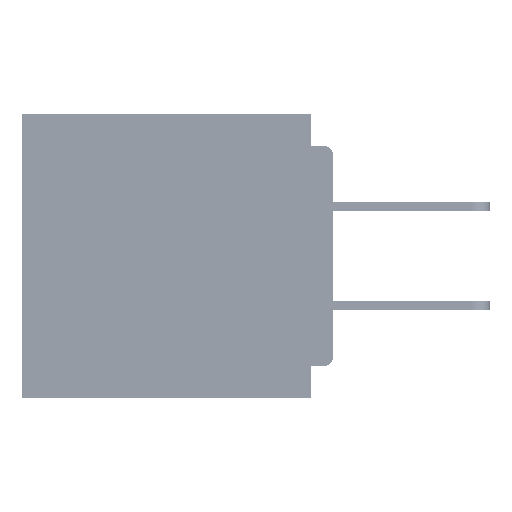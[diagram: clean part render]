
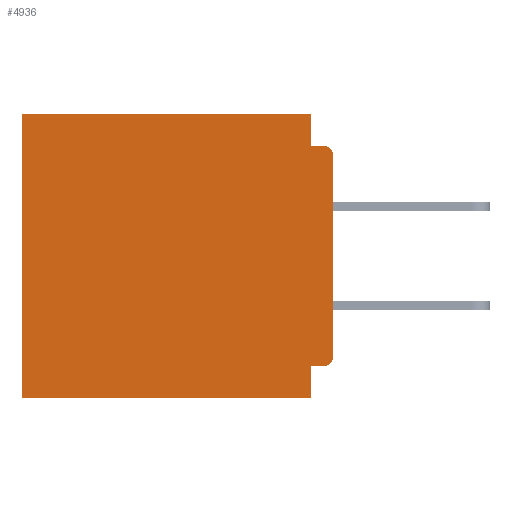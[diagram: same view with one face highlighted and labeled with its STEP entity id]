
A CAD part, left-side view. The second image highlights one B-rep face of the part: STEP entity #4936.
In plain terms, the highlighted planar face has unit normal (-1, 0, 0).
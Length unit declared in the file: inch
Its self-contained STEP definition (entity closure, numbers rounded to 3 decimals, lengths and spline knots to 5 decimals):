
#6 = ORIENTED_EDGE ( 'NONE', *, *, #24385, .F. ) ;
#186 = VERTEX_POINT ( 'NONE', #56536 ) ;
#1119 = VERTEX_POINT ( 'NONE', #56077 ) ;
#1601 = FACE_OUTER_BOUND ( 'NONE', #58669, .T. ) ;
#1822 = VERTEX_POINT ( 'NONE', #17377 ) ;
#1974 = PLANE ( 'NONE',  #14499 ) ;
#2165 = ORIENTED_EDGE ( 'NONE', *, *, #49622, .T. ) ;
#2526 = ORIENTED_EDGE ( 'NONE', *, *, #40947, .F. ) ;
#3678 = CARTESIAN_POINT ( 'NONE',  ( 0.3, 0., 0. ) ) ;
#3712 = AXIS2_PLACEMENT_3D ( 'NONE', #49629, #21771, #54325 ) ;
#3811 = CIRCLE ( 'NONE', #28204, 0.015 ) ;
#4936 = ADVANCED_FACE ( 'NONE', ( #1601 ), #1974, .F. ) ;
#5066 = VERTEX_POINT ( 'NONE', #24203 ) ;
#5212 = VECTOR ( 'NONE', #17366, 39.37008 ) ;
#7191 = ORIENTED_EDGE ( 'NONE', *, *, #28212, .F. ) ;
#7407 = CARTESIAN_POINT ( 'NONE',  ( 0.3, 0.437, 0. ) ) ;
#7862 = DIRECTION ( 'NONE',  ( 0., -1., 0. ) ) ;
#8269 = EDGE_CURVE ( 'NONE', #5066, #24304, #17191, .T. ) ;
#10052 = CIRCLE ( 'NONE', #3712, 0.015 ) ;
#11329 = DIRECTION ( 'NONE',  ( 1., 0., 0. ) ) ;
#12685 = DIRECTION ( 'NONE',  ( -1., 0., 0. ) ) ;
#14499 = AXIS2_PLACEMENT_3D ( 'NONE', #39167, #11329, #43852 ) ;
#16113 = VERTEX_POINT ( 'NONE', #37213 ) ;
#17191 = LINE ( 'NONE', #3678, #52838 ) ;
#17366 = DIRECTION ( 'NONE',  ( 0., 0., -1. ) ) ;
#17377 = CARTESIAN_POINT ( 'NONE',  ( 0.3, 0.031, -0.355 ) ) ;
#17601 = EDGE_CURVE ( 'NONE', #5066, #1119, #39386, .T. ) ;
#17845 = CARTESIAN_POINT ( 'NONE',  ( 0.3, 0., -0.4 ) ) ;
#18385 = VECTOR ( 'NONE', #50360, 39.37008 ) ;
#18921 = CARTESIAN_POINT ( 'NONE',  ( 0.3, 0.437, -0.4 ) ) ;
#19034 = LINE ( 'NONE', #22015, #5212 ) ;
#19107 = LINE ( 'NONE', #21187, #29941 ) ;
#20383 = ORIENTED_EDGE ( 'NONE', *, *, #23775, .F. ) ;
#21187 = CARTESIAN_POINT ( 'NONE',  ( 0.3, 0.437, -0.4 ) ) ;
#21771 = DIRECTION ( 'NONE',  ( -1., 0., 0. ) ) ;
#22015 = CARTESIAN_POINT ( 'NONE',  ( 0.3, 0., -0.4 ) ) ;
#23077 = DIRECTION ( 'NONE',  ( 0., 0., -1. ) ) ;
#23775 = EDGE_CURVE ( 'NONE', #16113, #25872, #40204, .T. ) ;
#24203 = CARTESIAN_POINT ( 'NONE',  ( 0.3, 0.031, 0. ) ) ;
#24304 = VERTEX_POINT ( 'NONE', #7407 ) ;
#24385 = EDGE_CURVE ( 'NONE', #45454, #46795, #19034, .T. ) ;
#25625 = CARTESIAN_POINT ( 'NONE',  ( 0.3, 0., -0.34 ) ) ;
#25872 = VERTEX_POINT ( 'NONE', #18921 ) ;
#27765 = CARTESIAN_POINT ( 'NONE',  ( 0.3, 0.015, -0.355 ) ) ;
#28204 = AXIS2_PLACEMENT_3D ( 'NONE', #40528, #12685, #45212 ) ;
#28212 = EDGE_CURVE ( 'NONE', #1822, #16113, #38984, .T. ) ;
#29413 = DIRECTION ( 'NONE',  ( 0., 0., -1. ) ) ;
#29941 = VECTOR ( 'NONE', #23077, 39.37008 ) ;
#30906 = EDGE_CURVE ( 'NONE', #47703, #46795, #3811, .T. ) ;
#31175 = ORIENTED_EDGE ( 'NONE', *, *, #45833, .T. ) ;
#33935 = CARTESIAN_POINT ( 'NONE',  ( 0.3, 0., -0.355 ) ) ;
#34951 = EDGE_CURVE ( 'NONE', #47703, #1822, #52752, .T. ) ;
#35737 = CARTESIAN_POINT ( 'NONE',  ( 0.3, 0., -0.045 ) ) ;
#37213 = CARTESIAN_POINT ( 'NONE',  ( 0.3, 0.031, -0.4 ) ) ;
#37937 = VECTOR ( 'NONE', #38262, 39.37008 ) ;
#38262 = DIRECTION ( 'NONE',  ( 0., 0., -1. ) ) ;
#38644 = DIRECTION ( 'NONE',  ( 0., 1., 0. ) ) ;
#38903 = VECTOR ( 'NONE', #38644, 39.37008 ) ;
#38984 = LINE ( 'NONE', #57310, #51379 ) ;
#39167 = CARTESIAN_POINT ( 'NONE',  ( 0.3, 0., -0.4 ) ) ;
#39386 = LINE ( 'NONE', #42941, #37937 ) ;
#40204 = LINE ( 'NONE', #17845, #18385 ) ;
#40528 = CARTESIAN_POINT ( 'NONE',  ( 0.3, 0.015, -0.34 ) ) ;
#40947 = EDGE_CURVE ( 'NONE', #1119, #186, #55364, .T. ) ;
#42941 = CARTESIAN_POINT ( 'NONE',  ( 0.3, 0.031, 0. ) ) ;
#43309 = CARTESIAN_POINT ( 'NONE',  ( 0.3, 0., -0.06 ) ) ;
#43852 = DIRECTION ( 'NONE',  ( 0., 0., -1. ) ) ;
#45212 = DIRECTION ( 'NONE',  ( 0., 0., -1. ) ) ;
#45454 = VERTEX_POINT ( 'NONE', #43309 ) ;
#45833 = EDGE_CURVE ( 'NONE', #24304, #25872, #19107, .T. ) ;
#46795 = VERTEX_POINT ( 'NONE', #25625 ) ;
#47703 = VERTEX_POINT ( 'NONE', #27765 ) ;
#48325 = ORIENTED_EDGE ( 'NONE', *, *, #17601, .F. ) ;
#49348 = ORIENTED_EDGE ( 'NONE', *, *, #34951, .F. ) ;
#49622 = EDGE_CURVE ( 'NONE', #45454, #186, #10052, .T. ) ;
#49629 = CARTESIAN_POINT ( 'NONE',  ( 0.3, 0.015, -0.06 ) ) ;
#49793 = ORIENTED_EDGE ( 'NONE', *, *, #30906, .T. ) ;
#50360 = DIRECTION ( 'NONE',  ( 0., 1., 0. ) ) ;
#51379 = VECTOR ( 'NONE', #29413, 39.37008 ) ;
#52752 = LINE ( 'NONE', #33935, #38903 ) ;
#52838 = VECTOR ( 'NONE', #59519, 39.37008 ) ;
#54325 = DIRECTION ( 'NONE',  ( 0., 0., -1. ) ) ;
#54336 = ORIENTED_EDGE ( 'NONE', *, *, #8269, .T. ) ;
#55364 = LINE ( 'NONE', #35737, #56818 ) ;
#56077 = CARTESIAN_POINT ( 'NONE',  ( 0.3, 0.031, -0.045 ) ) ;
#56536 = CARTESIAN_POINT ( 'NONE',  ( 0.3, 0.015, -0.045 ) ) ;
#56818 = VECTOR ( 'NONE', #7862, 39.37008 ) ;
#57310 = CARTESIAN_POINT ( 'NONE',  ( 0.3, 0.031, -0.4 ) ) ;
#58669 = EDGE_LOOP ( 'NONE', ( #6, #2165, #2526, #48325, #54336, #31175, #20383, #7191, #49348, #49793 ) ) ;
#59519 = DIRECTION ( 'NONE',  ( 0., 1., 0. ) ) ;
